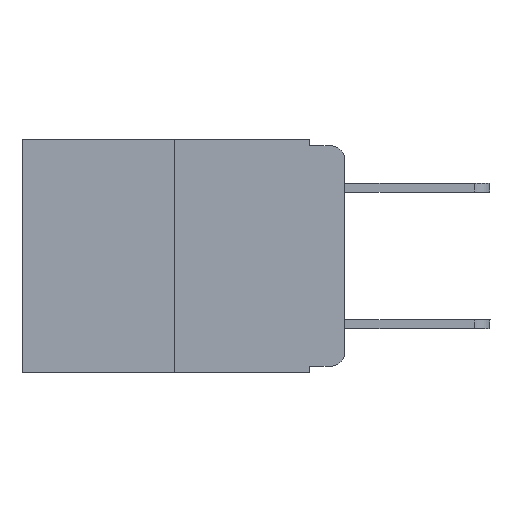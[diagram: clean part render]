
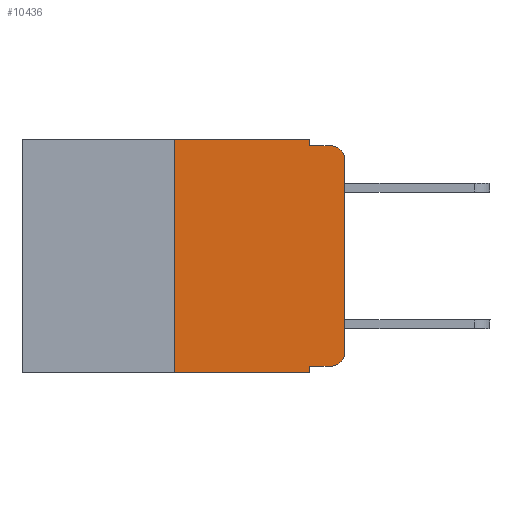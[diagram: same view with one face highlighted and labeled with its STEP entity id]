
A CAD part, left-side view. The second image highlights one B-rep face of the part: STEP entity #10436.
In plain terms, the highlighted planar face has unit normal (-1, 0, 0).
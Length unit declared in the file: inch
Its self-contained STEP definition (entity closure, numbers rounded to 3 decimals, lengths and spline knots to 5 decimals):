
#65 = DIRECTION ( 'NONE',  ( 0., -1., 0. ) ) ;
#111 = CARTESIAN_POINT ( 'NONE',  ( 0., 0.051, -0.333 ) ) ;
#187 = VERTEX_POINT ( 'NONE', #1609 ) ;
#557 = EDGE_CURVE ( 'NONE', #12142, #187, #12243, .T. ) ;
#927 = DIRECTION ( 'NONE',  ( -1., 0., 0. ) ) ;
#983 = VECTOR ( 'NONE', #1257, 39.37008 ) ;
#1064 = ORIENTED_EDGE ( 'NONE', *, *, #4534, .F. ) ;
#1257 = DIRECTION ( 'NONE',  ( 0., -1., 0. ) ) ;
#1261 = LINE ( 'NONE', #5821, #14104 ) ;
#1315 = DIRECTION ( 'NONE',  ( 0., 0., -1. ) ) ;
#1541 = CIRCLE ( 'NONE', #2847, 0.02 ) ;
#1609 = CARTESIAN_POINT ( 'NONE',  ( 0., 0., -0.313 ) ) ;
#1792 = CARTESIAN_POINT ( 'NONE',  ( 0., 0.051, -0.01 ) ) ;
#1889 = DIRECTION ( 'NONE',  ( 0., 0., -1. ) ) ;
#2119 = EDGE_CURVE ( 'NONE', #4876, #12653, #8117, .T. ) ;
#2175 = CARTESIAN_POINT ( 'NONE',  ( 0., 0.051, -0.01 ) ) ;
#2581 = VERTEX_POINT ( 'NONE', #1792 ) ;
#2613 = LINE ( 'NONE', #111, #7644 ) ;
#2847 = AXIS2_PLACEMENT_3D ( 'NONE', #3648, #11609, #8186 ) ;
#3329 = EDGE_CURVE ( 'NONE', #7684, #12142, #2613, .T. ) ;
#3525 = CARTESIAN_POINT ( 'NONE',  ( 0., 0.473, 0. ) ) ;
#3648 = CARTESIAN_POINT ( 'NONE',  ( 0., 0.02, -0.03 ) ) ;
#3728 = LINE ( 'NONE', #11185, #12990 ) ;
#3778 = ORIENTED_EDGE ( 'NONE', *, *, #9737, .F. ) ;
#3886 = CARTESIAN_POINT ( 'NONE',  ( 0., 0.051, 0. ) ) ;
#4213 = CARTESIAN_POINT ( 'NONE',  ( 0., 0.051, -0.333 ) ) ;
#4258 = CARTESIAN_POINT ( 'NONE',  ( 0., 0.25, 0. ) ) ;
#4534 = EDGE_CURVE ( 'NONE', #7684, #12653, #1261, .T. ) ;
#4567 = CARTESIAN_POINT ( 'NONE',  ( 0., 0., -0.03 ) ) ;
#4604 = LINE ( 'NONE', #8069, #5682 ) ;
#4660 = ORIENTED_EDGE ( 'NONE', *, *, #13171, .F. ) ;
#4876 = VERTEX_POINT ( 'NONE', #13197 ) ;
#5401 = ORIENTED_EDGE ( 'NONE', *, *, #557, .T. ) ;
#5682 = VECTOR ( 'NONE', #5844, 39.37008 ) ;
#5821 = CARTESIAN_POINT ( 'NONE',  ( 0., 0.051, 0. ) ) ;
#5844 = DIRECTION ( 'NONE',  ( 0., 0., -1. ) ) ;
#5912 = VERTEX_POINT ( 'NONE', #4258 ) ;
#6550 = DIRECTION ( 'NONE',  ( 0., 0., 1. ) ) ;
#6720 = ORIENTED_EDGE ( 'NONE', *, *, #7145, .T. ) ;
#6756 = DIRECTION ( 'NONE',  ( 0., -1., 0. ) ) ;
#6802 = DIRECTION ( 'NONE',  ( 0., 0., 1. ) ) ;
#7023 = PLANE ( 'NONE',  #12031 ) ;
#7065 = DIRECTION ( 'NONE',  ( 0., 0., -1. ) ) ;
#7145 = EDGE_CURVE ( 'NONE', #187, #12525, #3728, .T. ) ;
#7345 = FACE_OUTER_BOUND ( 'NONE', #11889, .T. ) ;
#7644 = VECTOR ( 'NONE', #65, 39.37008 ) ;
#7684 = VERTEX_POINT ( 'NONE', #4213 ) ;
#8069 = CARTESIAN_POINT ( 'NONE',  ( 0., 0.051, 0. ) ) ;
#8084 = EDGE_CURVE ( 'NONE', #12525, #13953, #1541, .T. ) ;
#8117 = LINE ( 'NONE', #8882, #13276 ) ;
#8186 = DIRECTION ( 'NONE',  ( 0., 0., -1. ) ) ;
#8589 = EDGE_CURVE ( 'NONE', #5912, #10023, #11693, .T. ) ;
#8833 = CARTESIAN_POINT ( 'NONE',  ( 0., 0.02, -0.313 ) ) ;
#8882 = CARTESIAN_POINT ( 'NONE',  ( 0., 0.473, -0.343 ) ) ;
#9026 = DIRECTION ( 'NONE',  ( 0., -1., 0. ) ) ;
#9737 = EDGE_CURVE ( 'NONE', #2581, #13953, #11484, .T. ) ;
#9891 = LINE ( 'NONE', #12399, #13277 ) ;
#10023 = VERTEX_POINT ( 'NONE', #3886 ) ;
#10333 = CARTESIAN_POINT ( 'NONE',  ( 0., 0.473, 0. ) ) ;
#10418 = CARTESIAN_POINT ( 'NONE',  ( 0., 0.051, -0.343 ) ) ;
#10436 = ADVANCED_FACE ( 'NONE', ( #7345 ), #7023, .F. ) ;
#10619 = ORIENTED_EDGE ( 'NONE', *, *, #2119, .T. ) ;
#10674 = CARTESIAN_POINT ( 'NONE',  ( 0., 0.02, -0.01 ) ) ;
#10725 = ORIENTED_EDGE ( 'NONE', *, *, #14448, .F. ) ;
#11185 = CARTESIAN_POINT ( 'NONE',  ( 0., 0., 0. ) ) ;
#11298 = ORIENTED_EDGE ( 'NONE', *, *, #8084, .T. ) ;
#11432 = DIRECTION ( 'NONE',  ( 1., 0., 0. ) ) ;
#11484 = LINE ( 'NONE', #2175, #14320 ) ;
#11609 = DIRECTION ( 'NONE',  ( -1., 0., 0. ) ) ;
#11693 = LINE ( 'NONE', #10333, #983 ) ;
#11889 = EDGE_LOOP ( 'NONE', ( #6720, #11298, #3778, #4660, #12930, #10725, #10619, #1064, #12913, #5401 ) ) ;
#12031 = AXIS2_PLACEMENT_3D ( 'NONE', #3525, #11432, #1315 ) ;
#12142 = VERTEX_POINT ( 'NONE', #12763 ) ;
#12243 = CIRCLE ( 'NONE', #14601, 0.02 ) ;
#12399 = CARTESIAN_POINT ( 'NONE',  ( 0., 0.25, 0. ) ) ;
#12525 = VERTEX_POINT ( 'NONE', #4567 ) ;
#12653 = VERTEX_POINT ( 'NONE', #10418 ) ;
#12763 = CARTESIAN_POINT ( 'NONE',  ( 0., 0.02, -0.333 ) ) ;
#12913 = ORIENTED_EDGE ( 'NONE', *, *, #3329, .T. ) ;
#12930 = ORIENTED_EDGE ( 'NONE', *, *, #8589, .F. ) ;
#12990 = VECTOR ( 'NONE', #6550, 39.37008 ) ;
#13171 = EDGE_CURVE ( 'NONE', #10023, #2581, #4604, .T. ) ;
#13197 = CARTESIAN_POINT ( 'NONE',  ( 0., 0.25, -0.343 ) ) ;
#13276 = VECTOR ( 'NONE', #6756, 39.37008 ) ;
#13277 = VECTOR ( 'NONE', #6802, 39.37008 ) ;
#13953 = VERTEX_POINT ( 'NONE', #10674 ) ;
#14104 = VECTOR ( 'NONE', #7065, 39.37008 ) ;
#14320 = VECTOR ( 'NONE', #9026, 39.37008 ) ;
#14448 = EDGE_CURVE ( 'NONE', #4876, #5912, #9891, .T. ) ;
#14601 = AXIS2_PLACEMENT_3D ( 'NONE', #8833, #927, #1889 ) ;
